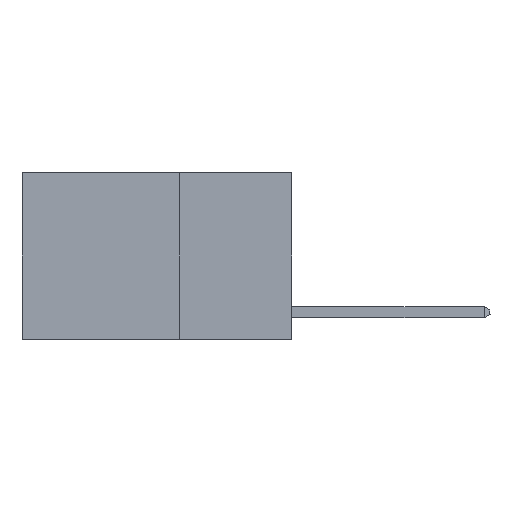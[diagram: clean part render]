
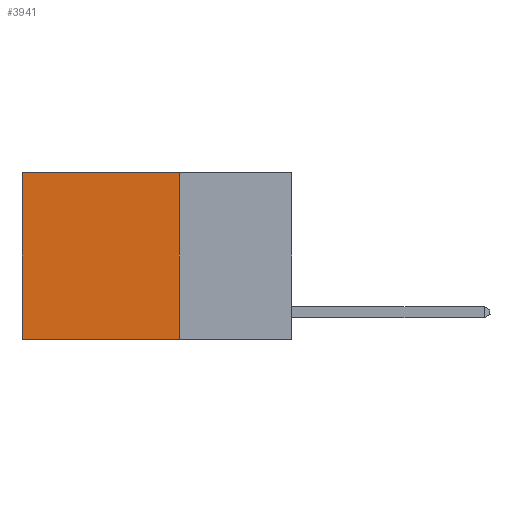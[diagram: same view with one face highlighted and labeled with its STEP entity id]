
A CAD part, left-side view. The second image highlights one B-rep face of the part: STEP entity #3941.
In plain terms, the highlighted planar face has unit normal (-1, 0, 0).
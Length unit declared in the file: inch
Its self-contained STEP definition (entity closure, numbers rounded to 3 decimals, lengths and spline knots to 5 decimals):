
#700 = ORIENTED_EDGE ( 'NONE', *, *, #5928, .T. ) ;
#1586 = CARTESIAN_POINT ( 'NONE',  ( 0.2625, 0.6, -0.37 ) ) ;
#2782 = CARTESIAN_POINT ( 'NONE',  ( 0.2625, 0.25, -0.37 ) ) ;
#3684 = CARTESIAN_POINT ( 'NONE',  ( 0.2625, 0.25, -0.37 ) ) ;
#3754 = ORIENTED_EDGE ( 'NONE', *, *, #24425, .T. ) ;
#3941 = ADVANCED_FACE ( 'NONE', ( #11424 ), #9407, .F. ) ;
#4173 = VERTEX_POINT ( 'NONE', #23615 ) ;
#5167 = VECTOR ( 'NONE', #8893, 39.37008 ) ;
#5449 = DIRECTION ( 'NONE',  ( 0., 0., -1. ) ) ;
#5538 = VECTOR ( 'NONE', #14567, 39.37008 ) ;
#5609 = LINE ( 'NONE', #3684, #6007 ) ;
#5697 = CARTESIAN_POINT ( 'NONE',  ( 0.2625, 0.25, 0. ) ) ;
#5928 = EDGE_CURVE ( 'NONE', #23946, #12628, #11048, .T. ) ;
#6007 = VECTOR ( 'NONE', #7636, 39.37008 ) ;
#6794 = CARTESIAN_POINT ( 'NONE',  ( 0.2625, 0.25, 0. ) ) ;
#7636 = DIRECTION ( 'NONE',  ( 0., 1., 0. ) ) ;
#8485 = EDGE_LOOP ( 'NONE', ( #700, #11254, #10131, #3754 ) ) ;
#8780 = AXIS2_PLACEMENT_3D ( 'NONE', #5697, #13235, #5449 ) ;
#8893 = DIRECTION ( 'NONE',  ( 0., 0., -1. ) ) ;
#9407 = PLANE ( 'NONE',  #8780 ) ;
#10131 = ORIENTED_EDGE ( 'NONE', *, *, #13049, .F. ) ;
#10193 = VECTOR ( 'NONE', #18871, 39.37008 ) ;
#11048 = LINE ( 'NONE', #20458, #5167 ) ;
#11254 = ORIENTED_EDGE ( 'NONE', *, *, #13673, .F. ) ;
#11424 = FACE_OUTER_BOUND ( 'NONE', #8485, .T. ) ;
#12628 = VERTEX_POINT ( 'NONE', #1586 ) ;
#13049 = EDGE_CURVE ( 'NONE', #4173, #13373, #24214, .T. ) ;
#13235 = DIRECTION ( 'NONE',  ( 1., 0., 0. ) ) ;
#13373 = VERTEX_POINT ( 'NONE', #2782 ) ;
#13673 = EDGE_CURVE ( 'NONE', #13373, #12628, #5609, .T. ) ;
#14567 = DIRECTION ( 'NONE',  ( 0., 0., -1. ) ) ;
#14806 = CARTESIAN_POINT ( 'NONE',  ( 0.2625, 0.6, 0. ) ) ;
#15394 = LINE ( 'NONE', #19448, #10193 ) ;
#18871 = DIRECTION ( 'NONE',  ( 0., 1., 0. ) ) ;
#19448 = CARTESIAN_POINT ( 'NONE',  ( 0.2625, 0.25, 0. ) ) ;
#20458 = CARTESIAN_POINT ( 'NONE',  ( 0.2625, 0.6, 0. ) ) ;
#23615 = CARTESIAN_POINT ( 'NONE',  ( 0.2625, 0.25, 0. ) ) ;
#23946 = VERTEX_POINT ( 'NONE', #14806 ) ;
#24214 = LINE ( 'NONE', #6794, #5538 ) ;
#24425 = EDGE_CURVE ( 'NONE', #4173, #23946, #15394, .T. ) ;
